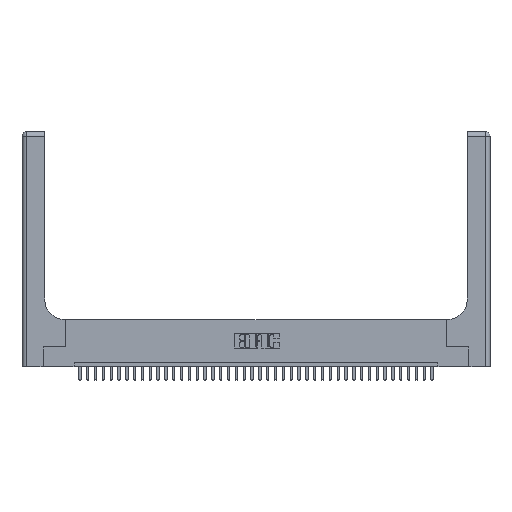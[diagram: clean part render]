
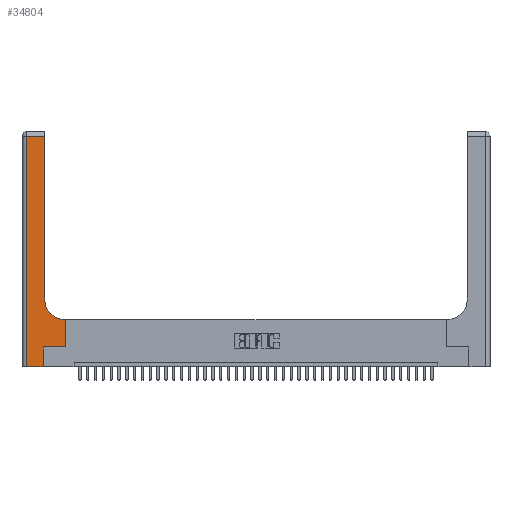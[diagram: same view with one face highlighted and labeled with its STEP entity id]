
A CAD part, top view. The second image highlights one B-rep face of the part: STEP entity #34804.
In plain terms, the highlighted planar face has unit normal (0, 0, 1).
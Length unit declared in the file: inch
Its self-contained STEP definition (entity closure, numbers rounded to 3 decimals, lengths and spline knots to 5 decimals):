
#77 = VECTOR ( 'NONE', #32309, 39.37008 ) ;
#248 = ORIENTED_EDGE ( 'NONE', *, *, #20350, .T. ) ;
#455 = CARTESIAN_POINT ( 'NONE',  ( 0.5585, 0.6, 0.37 ) ) ;
#577 = EDGE_CURVE ( 'NONE', #36495, #37002, #34465, .T. ) ;
#1016 = ORIENTED_EDGE ( 'NONE', *, *, #20689, .T. ) ;
#1203 = PLANE ( 'NONE',  #1297 ) ;
#1297 = AXIS2_PLACEMENT_3D ( 'NONE', #7618, #10937, #37891 ) ;
#3441 = CARTESIAN_POINT ( 'NONE',  ( 0.2915, 2.94, 0.37 ) ) ;
#4418 = CARTESIAN_POINT ( 'NONE',  ( 0.269, 0.25, 0.37 ) ) ;
#5201 = ORIENTED_EDGE ( 'NONE', *, *, #14777, .T. ) ;
#5817 = LINE ( 'NONE', #11002, #8195 ) ;
#6626 = CARTESIAN_POINT ( 'NONE',  ( 0.06, 3., 0.37 ) ) ;
#7533 = EDGE_CURVE ( 'NONE', #24040, #36495, #28890, .T. ) ;
#7618 = CARTESIAN_POINT ( 'NONE',  ( 0., 3., 0.37 ) ) ;
#8137 = DIRECTION ( 'NONE',  ( 0., -1., 0. ) ) ;
#8195 = VECTOR ( 'NONE', #14198, 39.37008 ) ;
#8284 = CARTESIAN_POINT ( 'NONE',  ( 0., 2.94, 0.37 ) ) ;
#10035 = CARTESIAN_POINT ( 'NONE',  ( 0.06, 2.94, 0.37 ) ) ;
#10594 = CARTESIAN_POINT ( 'NONE',  ( 0.5415, 0.6, 0.37 ) ) ;
#10684 = VECTOR ( 'NONE', #31690, 39.37008 ) ;
#10937 = DIRECTION ( 'NONE',  ( 0., 0., -1. ) ) ;
#11002 = CARTESIAN_POINT ( 'NONE',  ( 0.269, 0., 0.37 ) ) ;
#11079 = DIRECTION ( 'NONE',  ( 0., 0., -1. ) ) ;
#12732 = VECTOR ( 'NONE', #8137, 39.37008 ) ;
#13031 = CARTESIAN_POINT ( 'NONE',  ( 0.2915, 0.6, 0.37 ) ) ;
#14081 = VECTOR ( 'NONE', #22621, 39.37008 ) ;
#14137 = DIRECTION ( 'NONE',  ( 1., 0., 0. ) ) ;
#14198 = DIRECTION ( 'NONE',  ( 0., 1., 0. ) ) ;
#14471 = CARTESIAN_POINT ( 'NONE',  ( 0.2915, 3., 0.37 ) ) ;
#14668 = VERTEX_POINT ( 'NONE', #10035 ) ;
#14777 = EDGE_CURVE ( 'NONE', #35309, #24040, #38180, .T. ) ;
#15121 = ORIENTED_EDGE ( 'NONE', *, *, #15305, .T. ) ;
#15305 = EDGE_CURVE ( 'NONE', #33487, #26077, #5817, .T. ) ;
#17309 = VERTEX_POINT ( 'NONE', #20305 ) ;
#17438 = ORIENTED_EDGE ( 'NONE', *, *, #31772, .T. ) ;
#17949 = VERTEX_POINT ( 'NONE', #25291 ) ;
#18144 = LINE ( 'NONE', #37816, #32415 ) ;
#19451 = CARTESIAN_POINT ( 'NONE',  ( 0.2915, 0.85, 0.37 ) ) ;
#20305 = CARTESIAN_POINT ( 'NONE',  ( 0.06, 0., 0.37 ) ) ;
#20350 = EDGE_CURVE ( 'NONE', #17309, #33487, #37233, .T. ) ;
#20689 = EDGE_CURVE ( 'NONE', #26077, #17949, #24509, .T. ) ;
#20846 = DIRECTION ( 'NONE',  ( -1., 0., 0. ) ) ;
#22252 = EDGE_CURVE ( 'NONE', #37002, #14668, #32424, .T. ) ;
#22328 = CARTESIAN_POINT ( 'NONE',  ( 0.269, 0., 0.37 ) ) ;
#22430 = DIRECTION ( 'NONE',  ( 0., 1., 0. ) ) ;
#22525 = VECTOR ( 'NONE', #20846, 39.37008 ) ;
#22621 = DIRECTION ( 'NONE',  ( 1., 0., 0. ) ) ;
#24040 = VERTEX_POINT ( 'NONE', #10594 ) ;
#24509 = LINE ( 'NONE', #31745, #14081 ) ;
#25291 = CARTESIAN_POINT ( 'NONE',  ( 0.5585, 0.25, 0.37 ) ) ;
#26077 = VERTEX_POINT ( 'NONE', #4418 ) ;
#26693 = FACE_OUTER_BOUND ( 'NONE', #35805, .T. ) ;
#28504 = AXIS2_PLACEMENT_3D ( 'NONE', #32039, #11079, #14137 ) ;
#28890 = CIRCLE ( 'NONE', #28504, 0.25 ) ;
#29526 = ORIENTED_EDGE ( 'NONE', *, *, #577, .T. ) ;
#30273 = EDGE_CURVE ( 'NONE', #17949, #35309, #18144, .T. ) ;
#30628 = ORIENTED_EDGE ( 'NONE', *, *, #7533, .T. ) ;
#31690 = DIRECTION ( 'NONE',  ( 1., 0., 0. ) ) ;
#31745 = CARTESIAN_POINT ( 'NONE',  ( 0.269, 0.25, 0.37 ) ) ;
#31772 = EDGE_CURVE ( 'NONE', #14668, #17309, #31782, .T. ) ;
#31782 = LINE ( 'NONE', #6626, #12732 ) ;
#32039 = CARTESIAN_POINT ( 'NONE',  ( 0.5415, 0.85, 0.37 ) ) ;
#32309 = DIRECTION ( 'NONE',  ( -1., 0., 0. ) ) ;
#32415 = VECTOR ( 'NONE', #22430, 39.37008 ) ;
#32424 = LINE ( 'NONE', #8284, #77 ) ;
#32552 = ORIENTED_EDGE ( 'NONE', *, *, #22252, .T. ) ;
#32777 = ORIENTED_EDGE ( 'NONE', *, *, #30273, .T. ) ;
#33487 = VERTEX_POINT ( 'NONE', #22328 ) ;
#34465 = LINE ( 'NONE', #14471, #37798 ) ;
#34804 = ADVANCED_FACE ( 'NONE', ( #26693 ), #1203, .F. ) ;
#35309 = VERTEX_POINT ( 'NONE', #455 ) ;
#35805 = EDGE_LOOP ( 'NONE', ( #29526, #32552, #17438, #248, #15121, #1016, #32777, #5201, #30628 ) ) ;
#36495 = VERTEX_POINT ( 'NONE', #19451 ) ;
#37002 = VERTEX_POINT ( 'NONE', #3441 ) ;
#37233 = LINE ( 'NONE', #37526, #10684 ) ;
#37526 = CARTESIAN_POINT ( 'NONE',  ( 0., 0., 0.37 ) ) ;
#37798 = VECTOR ( 'NONE', #38894, 39.37008 ) ;
#37816 = CARTESIAN_POINT ( 'NONE',  ( 0.5585, 0.25, 0.37 ) ) ;
#37891 = DIRECTION ( 'NONE',  ( -1., 0., 0. ) ) ;
#38180 = LINE ( 'NONE', #13031, #22525 ) ;
#38894 = DIRECTION ( 'NONE',  ( 0., 1., 0. ) ) ;
